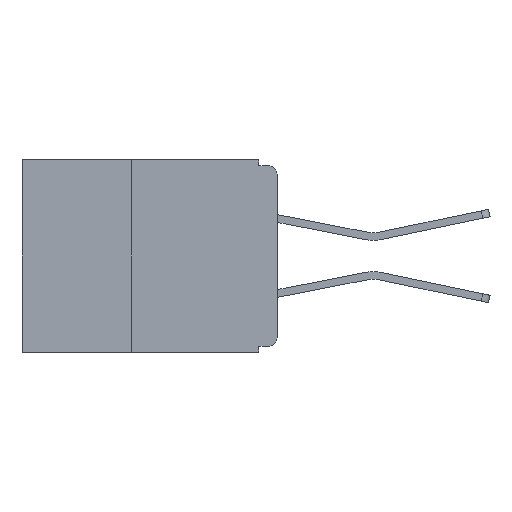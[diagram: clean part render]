
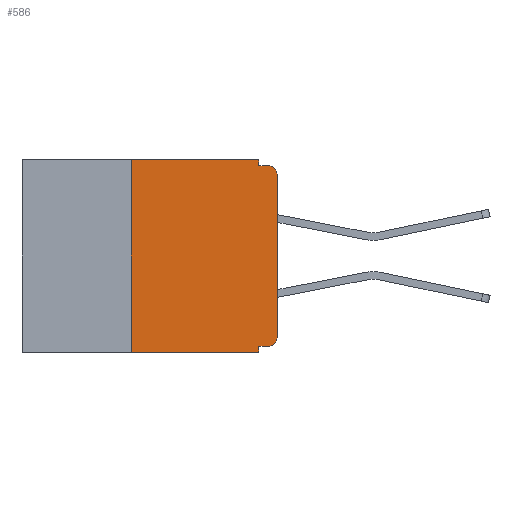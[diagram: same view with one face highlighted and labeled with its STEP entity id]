
A CAD part, left-side view. The second image highlights one B-rep face of the part: STEP entity #586.
In plain terms, the highlighted planar face has unit normal (-1, 0, 0).
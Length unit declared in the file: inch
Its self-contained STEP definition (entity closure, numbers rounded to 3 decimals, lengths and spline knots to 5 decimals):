
#4 = CIRCLE ( 'NONE', #867, 0.015 ) ;
#294 = VERTEX_POINT ( 'NONE', #12776 ) ;
#342 = EDGE_CURVE ( 'NONE', #5848, #8853, #5622, .T. ) ;
#517 = DIRECTION ( 'NONE',  ( 0., 0., -1. ) ) ;
#551 = LINE ( 'NONE', #11976, #590 ) ;
#585 = DIRECTION ( 'NONE',  ( 0., 0., 1. ) ) ;
#586 = ADVANCED_FACE ( 'NONE', ( #7455 ), #5339, .F. ) ;
#590 = VECTOR ( 'NONE', #11910, 39.37008 ) ;
#616 = CARTESIAN_POINT ( 'NONE',  ( 0., 0., 0. ) ) ;
#763 = CARTESIAN_POINT ( 'NONE',  ( 0., 0.25, -0.33 ) ) ;
#867 = AXIS2_PLACEMENT_3D ( 'NONE', #4189, #4132, #4071 ) ;
#1614 = AXIS2_PLACEMENT_3D ( 'NONE', #7435, #7330, #7297 ) ;
#1857 = EDGE_CURVE ( 'NONE', #5683, #5734, #10128, .T. ) ;
#2118 = CIRCLE ( 'NONE', #1614, 0.015 ) ;
#2275 = VECTOR ( 'NONE', #3661, 39.37008 ) ;
#2354 = LINE ( 'NONE', #3901, #2275 ) ;
#3413 = CARTESIAN_POINT ( 'NONE',  ( 0., 0.031, 0. ) ) ;
#3617 = ORIENTED_EDGE ( 'NONE', *, *, #342, .F. ) ;
#3661 = DIRECTION ( 'NONE',  ( 0., 0., -1. ) ) ;
#3737 = ORIENTED_EDGE ( 'NONE', *, *, #9967, .F. ) ;
#3804 = EDGE_LOOP ( 'NONE', ( #3995, #4486, #5450, #11166, #3617, #5991, #6125, #8480, #3737, #10522 ) ) ;
#3901 = CARTESIAN_POINT ( 'NONE',  ( 0., 0.031, -0.33 ) ) ;
#3995 = ORIENTED_EDGE ( 'NONE', *, *, #13070, .T. ) ;
#4071 = DIRECTION ( 'NONE',  ( 0., 0., -1. ) ) ;
#4090 = DIRECTION ( 'NONE',  ( 0., -1., 0. ) ) ;
#4132 = DIRECTION ( 'NONE',  ( -1., 0., 0. ) ) ;
#4189 = CARTESIAN_POINT ( 'NONE',  ( 0., 0.015, -0.305 ) ) ;
#4408 = VERTEX_POINT ( 'NONE', #13056 ) ;
#4486 = ORIENTED_EDGE ( 'NONE', *, *, #12174, .T. ) ;
#5268 = DIRECTION ( 'NONE',  ( 1., 0., 0. ) ) ;
#5339 = PLANE ( 'NONE',  #9087 ) ;
#5416 = VECTOR ( 'NONE', #4090, 39.37008 ) ;
#5450 = ORIENTED_EDGE ( 'NONE', *, *, #1857, .F. ) ;
#5501 = VERTEX_POINT ( 'NONE', #12336 ) ;
#5511 = VECTOR ( 'NONE', #6959, 39.37008 ) ;
#5622 = LINE ( 'NONE', #11517, #5416 ) ;
#5683 = VERTEX_POINT ( 'NONE', #9631 ) ;
#5734 = VERTEX_POINT ( 'NONE', #8847 ) ;
#5848 = VERTEX_POINT ( 'NONE', #7477 ) ;
#5991 = ORIENTED_EDGE ( 'NONE', *, *, #12586, .F. ) ;
#6125 = ORIENTED_EDGE ( 'NONE', *, *, #12816, .T. ) ;
#6320 = LINE ( 'NONE', #6940, #5511 ) ;
#6569 = DIRECTION ( 'NONE',  ( 0., 1., 0. ) ) ;
#6860 = CARTESIAN_POINT ( 'NONE',  ( 0., 0., -0.32 ) ) ;
#6940 = CARTESIAN_POINT ( 'NONE',  ( 0., 0.437, -0.33 ) ) ;
#6959 = DIRECTION ( 'NONE',  ( 0., -1., 0. ) ) ;
#7263 = EDGE_CURVE ( 'NONE', #7836, #294, #4, .T. ) ;
#7297 = DIRECTION ( 'NONE',  ( 0., 0., -1. ) ) ;
#7330 = DIRECTION ( 'NONE',  ( -1., 0., 0. ) ) ;
#7435 = CARTESIAN_POINT ( 'NONE',  ( 0., 0.015, -0.025 ) ) ;
#7455 = FACE_OUTER_BOUND ( 'NONE', #3804, .T. ) ;
#7477 = CARTESIAN_POINT ( 'NONE',  ( 0., 0.25, 0. ) ) ;
#7836 = VERTEX_POINT ( 'NONE', #9790 ) ;
#8480 = ORIENTED_EDGE ( 'NONE', *, *, #12941, .F. ) ;
#8847 = CARTESIAN_POINT ( 'NONE',  ( 0., 0.015, -0.01 ) ) ;
#8853 = VERTEX_POINT ( 'NONE', #3413 ) ;
#8880 = VECTOR ( 'NONE', #9532, 39.37008 ) ;
#9087 = AXIS2_PLACEMENT_3D ( 'NONE', #12431, #5268, #517 ) ;
#9316 = CARTESIAN_POINT ( 'NONE',  ( 0., 0., -0.01 ) ) ;
#9524 = VERTEX_POINT ( 'NONE', #13379 ) ;
#9532 = DIRECTION ( 'NONE',  ( 0., -1., 0. ) ) ;
#9576 = VECTOR ( 'NONE', #10601, 39.37008 ) ;
#9631 = CARTESIAN_POINT ( 'NONE',  ( 0., 0.031, -0.01 ) ) ;
#9728 = LINE ( 'NONE', #10652, #9576 ) ;
#9790 = CARTESIAN_POINT ( 'NONE',  ( 0., 0.015, -0.32 ) ) ;
#9967 = EDGE_CURVE ( 'NONE', #7836, #9524, #10475, .T. ) ;
#10128 = LINE ( 'NONE', #9316, #8880 ) ;
#10395 = VERTEX_POINT ( 'NONE', #763 ) ;
#10444 = VECTOR ( 'NONE', #6569, 39.37008 ) ;
#10475 = LINE ( 'NONE', #6860, #10444 ) ;
#10522 = ORIENTED_EDGE ( 'NONE', *, *, #7263, .T. ) ;
#10601 = DIRECTION ( 'NONE',  ( 0., 0., 1. ) ) ;
#10652 = CARTESIAN_POINT ( 'NONE',  ( 0., 0.25, -0.33 ) ) ;
#10999 = VECTOR ( 'NONE', #585, 39.37008 ) ;
#11158 = LINE ( 'NONE', #616, #10999 ) ;
#11166 = ORIENTED_EDGE ( 'NONE', *, *, #12501, .F. ) ;
#11517 = CARTESIAN_POINT ( 'NONE',  ( 0., 0.437, 0. ) ) ;
#11910 = DIRECTION ( 'NONE',  ( 0., 0., -1. ) ) ;
#11976 = CARTESIAN_POINT ( 'NONE',  ( 0., 0.031, 0. ) ) ;
#12174 = EDGE_CURVE ( 'NONE', #5501, #5734, #2118, .T. ) ;
#12336 = CARTESIAN_POINT ( 'NONE',  ( 0., 0., -0.025 ) ) ;
#12431 = CARTESIAN_POINT ( 'NONE',  ( 0., 0.437, 0. ) ) ;
#12501 = EDGE_CURVE ( 'NONE', #8853, #5683, #551, .T. ) ;
#12586 = EDGE_CURVE ( 'NONE', #10395, #5848, #9728, .T. ) ;
#12776 = CARTESIAN_POINT ( 'NONE',  ( 0., 0., -0.305 ) ) ;
#12816 = EDGE_CURVE ( 'NONE', #10395, #4408, #6320, .T. ) ;
#12941 = EDGE_CURVE ( 'NONE', #9524, #4408, #2354, .T. ) ;
#13056 = CARTESIAN_POINT ( 'NONE',  ( 0., 0.031, -0.33 ) ) ;
#13070 = EDGE_CURVE ( 'NONE', #294, #5501, #11158, .T. ) ;
#13379 = CARTESIAN_POINT ( 'NONE',  ( 0., 0.031, -0.32 ) ) ;
